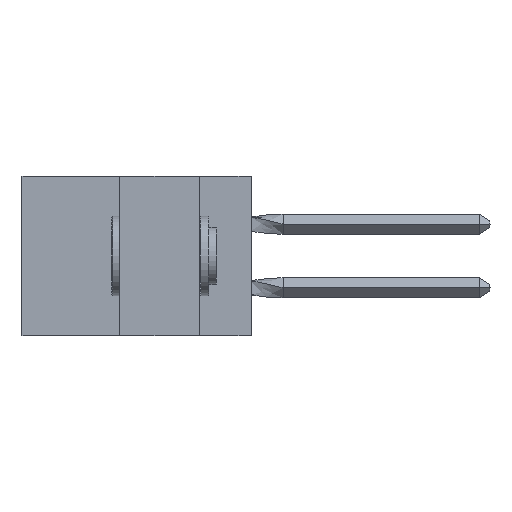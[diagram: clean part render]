
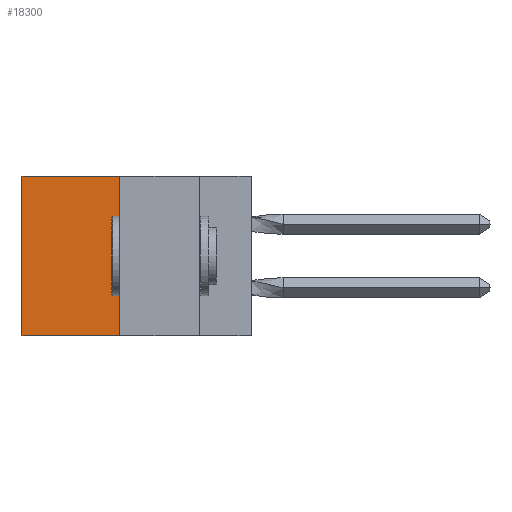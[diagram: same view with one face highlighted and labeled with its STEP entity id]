
A CAD part, left-side view. The second image highlights one B-rep face of the part: STEP entity #18300.
In plain terms, the highlighted planar face has unit normal (-1, 0, 0).
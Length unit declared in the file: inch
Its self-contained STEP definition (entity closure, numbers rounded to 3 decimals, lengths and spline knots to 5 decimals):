
#51 = CARTESIAN_POINT ( 'NONE',  ( 0.305, 0.413, -0.5 ) ) ;
#1078 = LINE ( 'NONE', #17663, #13432 ) ;
#2932 = CARTESIAN_POINT ( 'NONE',  ( 0.305, 0.72, 0. ) ) ;
#3453 = DIRECTION ( 'NONE',  ( 0., 1., 0. ) ) ;
#3535 = CARTESIAN_POINT ( 'NONE',  ( 0.305, 0.413, 0. ) ) ;
#3624 = EDGE_CURVE ( 'NONE', #13907, #15338, #10832, .T. ) ;
#3739 = VECTOR ( 'NONE', #9082, 39.37008 ) ;
#5008 = DIRECTION ( 'NONE',  ( 0., 1., 0. ) ) ;
#5554 = VERTEX_POINT ( 'NONE', #6127 ) ;
#5708 = AXIS2_PLACEMENT_3D ( 'NONE', #15871, #13194, #17537 ) ;
#6004 = ORIENTED_EDGE ( 'NONE', *, *, #9922, .F. ) ;
#6127 = CARTESIAN_POINT ( 'NONE',  ( 0.305, 0.72, -0.5 ) ) ;
#7600 = LINE ( 'NONE', #11870, #3739 ) ;
#8628 = VERTEX_POINT ( 'NONE', #2932 ) ;
#9082 = DIRECTION ( 'NONE',  ( 0., 0., -1. ) ) ;
#9922 = EDGE_CURVE ( 'NONE', #15338, #5554, #13190, .T. ) ;
#10108 = DIRECTION ( 'NONE',  ( 0., 0., -1. ) ) ;
#10798 = EDGE_CURVE ( 'NONE', #8628, #5554, #7600, .T. ) ;
#10832 = LINE ( 'NONE', #51, #17546 ) ;
#11051 = CARTESIAN_POINT ( 'NONE',  ( 0.305, 0.413, -0.5 ) ) ;
#11235 = FACE_OUTER_BOUND ( 'NONE', #11777, .T. ) ;
#11777 = EDGE_LOOP ( 'NONE', ( #15309, #6004, #12040, #17927 ) ) ;
#11870 = CARTESIAN_POINT ( 'NONE',  ( 0.305, 0.72, -0.5 ) ) ;
#12040 = ORIENTED_EDGE ( 'NONE', *, *, #3624, .F. ) ;
#12743 = VECTOR ( 'NONE', #5008, 39.37008 ) ;
#13190 = LINE ( 'NONE', #11051, #12743 ) ;
#13194 = DIRECTION ( 'NONE',  ( 1., 0., 0. ) ) ;
#13432 = VECTOR ( 'NONE', #3453, 39.37008 ) ;
#13907 = VERTEX_POINT ( 'NONE', #3535 ) ;
#14623 = CARTESIAN_POINT ( 'NONE',  ( 0.305, 0.413, -0.5 ) ) ;
#15309 = ORIENTED_EDGE ( 'NONE', *, *, #10798, .T. ) ;
#15338 = VERTEX_POINT ( 'NONE', #14623 ) ;
#15434 = EDGE_CURVE ( 'NONE', #13907, #8628, #1078, .T. ) ;
#15871 = CARTESIAN_POINT ( 'NONE',  ( 0.305, 0.413, -0.5 ) ) ;
#17342 = PLANE ( 'NONE',  #5708 ) ;
#17537 = DIRECTION ( 'NONE',  ( 0., 0., -1. ) ) ;
#17546 = VECTOR ( 'NONE', #10108, 39.37008 ) ;
#17663 = CARTESIAN_POINT ( 'NONE',  ( 0.305, 0.413, 0. ) ) ;
#17927 = ORIENTED_EDGE ( 'NONE', *, *, #15434, .T. ) ;
#18300 = ADVANCED_FACE ( 'NONE', ( #11235 ), #17342, .F. ) ;
